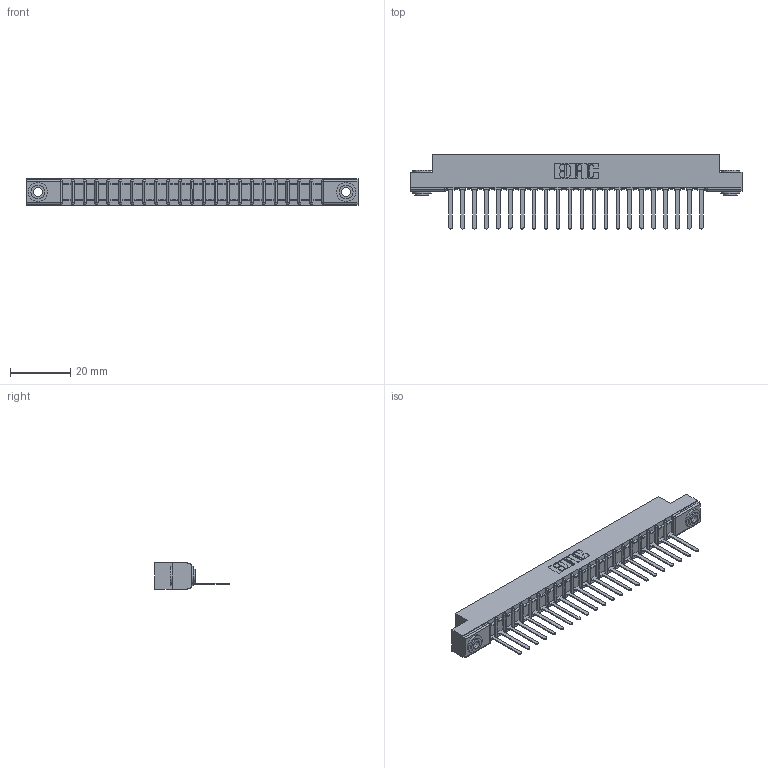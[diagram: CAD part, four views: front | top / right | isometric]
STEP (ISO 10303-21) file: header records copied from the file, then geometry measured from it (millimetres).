
FILE_DESCRIPTION (( 'STEP AP203' ), '1' );
FILE_NAME ('307-022-541-103.STEP', '2018-08-04T03:43:23', ( '' ), ( '' ), 'SwSTEP 2.0', 'SolidWorks 2016', '' );
FILE_SCHEMA (( 'CONFIG_CONTROL_DESIGN' ));
Length unit declared in the file: inch
Products named in the file (4): 307 Part_.156 Dia Mounting Holes; 307-290-002_541; 345-250-002_345-250-002-102; 307-022-541-103
Assembly tree (25 placements, depth 2):
  307-022-541-103
    307 Part_.156 Dia Mounting Holes
    307-290-002_541  x22
    345-250-002_345-250-002-102  x2
Bounding box: 110.19 x 24.59 x 8.71 mm (x, y, z)
Volume: 7337.6 mm3; surface area: 13964.7 mm2
Topology: 25 solids, 25 shells, 1821 faces, 5539 edges, 3626 vertices
Faces by surface type: plane 1084, cylinder 683, sphere 46, cone 8
Entity records: 23109 total; most frequent: CARTESIAN_POINT 3873, ORIENTED_EDGE 3854, DIRECTION 3787, EDGE_CURVE 1927, VECTOR 1459, LINE 1459, VERTEX_POINT 1250, AXIS2_PLACEMENT_3D 1164
